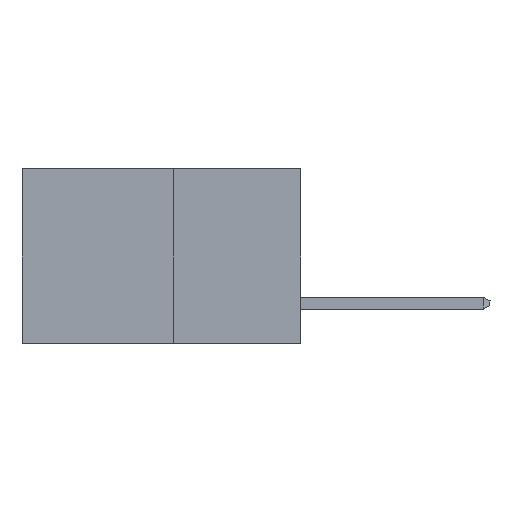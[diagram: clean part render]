
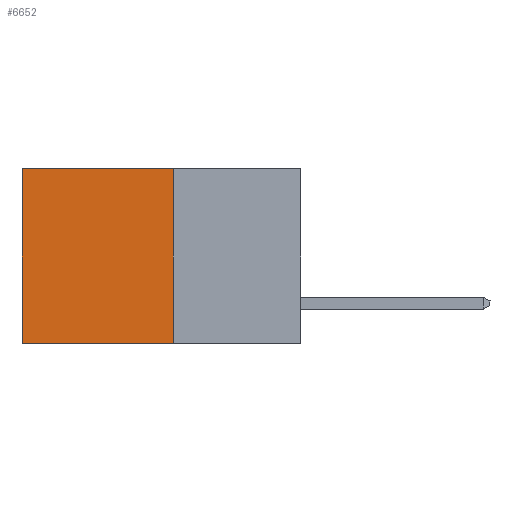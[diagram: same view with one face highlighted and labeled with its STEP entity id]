
A CAD part, left-side view. The second image highlights one B-rep face of the part: STEP entity #6652.
In plain terms, the highlighted planar face has unit normal (-1, 0, 0).
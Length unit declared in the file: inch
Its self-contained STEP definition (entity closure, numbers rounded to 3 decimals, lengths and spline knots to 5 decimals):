
#499 = ORIENTED_EDGE ( 'NONE', *, *, #7842, .T. ) ;
#1290 = DIRECTION ( 'NONE',  ( 0., 0., -1. ) ) ;
#1353 = EDGE_LOOP ( 'NONE', ( #499, #7801, #4283, #7589 ) ) ;
#1974 = LINE ( 'NONE', #6457, #2198 ) ;
#2198 = VECTOR ( 'NONE', #8405, 39.37008 ) ;
#2236 = DIRECTION ( 'NONE',  ( 1., 0., 0. ) ) ;
#2312 = DIRECTION ( 'NONE',  ( 0., 0., -1. ) ) ;
#2351 = LINE ( 'NONE', #6739, #5914 ) ;
#2553 = FACE_OUTER_BOUND ( 'NONE', #1353, .T. ) ;
#2642 = LINE ( 'NONE', #7510, #4272 ) ;
#3266 = EDGE_CURVE ( 'NONE', #6267, #3683, #5789, .T. ) ;
#3385 = CARTESIAN_POINT ( 'NONE',  ( 0.277, 0.59, -0.37 ) ) ;
#3669 = EDGE_CURVE ( 'NONE', #3683, #6469, #1974, .T. ) ;
#3683 = VERTEX_POINT ( 'NONE', #6424 ) ;
#4036 = VECTOR ( 'NONE', #1290, 39.37008 ) ;
#4272 = VECTOR ( 'NONE', #4903, 39.37008 ) ;
#4283 = ORIENTED_EDGE ( 'NONE', *, *, #3266, .F. ) ;
#4903 = DIRECTION ( 'NONE',  ( 0., 0., -1. ) ) ;
#5360 = AXIS2_PLACEMENT_3D ( 'NONE', #6224, #2236, #2312 ) ;
#5653 = CARTESIAN_POINT ( 'NONE',  ( 0.277, 0.27, -0.37 ) ) ;
#5789 = LINE ( 'NONE', #5653, #4036 ) ;
#5914 = VECTOR ( 'NONE', #6766, 39.37008 ) ;
#6224 = CARTESIAN_POINT ( 'NONE',  ( 0.277, 0.27, -0.37 ) ) ;
#6267 = VERTEX_POINT ( 'NONE', #7717 ) ;
#6354 = CARTESIAN_POINT ( 'NONE',  ( 0.277, 0.59, 0. ) ) ;
#6383 = VERTEX_POINT ( 'NONE', #6354 ) ;
#6424 = CARTESIAN_POINT ( 'NONE',  ( 0.277, 0.27, -0.37 ) ) ;
#6457 = CARTESIAN_POINT ( 'NONE',  ( 0.277, 0.27, -0.37 ) ) ;
#6469 = VERTEX_POINT ( 'NONE', #3385 ) ;
#6645 = PLANE ( 'NONE',  #5360 ) ;
#6652 = ADVANCED_FACE ( 'NONE', ( #2553 ), #6645, .F. ) ;
#6739 = CARTESIAN_POINT ( 'NONE',  ( 0.277, 0.27, 0. ) ) ;
#6766 = DIRECTION ( 'NONE',  ( 0., 1., 0. ) ) ;
#7510 = CARTESIAN_POINT ( 'NONE',  ( 0.277, 0.59, -0.37 ) ) ;
#7589 = ORIENTED_EDGE ( 'NONE', *, *, #8526, .T. ) ;
#7717 = CARTESIAN_POINT ( 'NONE',  ( 0.277, 0.27, 0. ) ) ;
#7801 = ORIENTED_EDGE ( 'NONE', *, *, #3669, .F. ) ;
#7842 = EDGE_CURVE ( 'NONE', #6383, #6469, #2642, .T. ) ;
#8405 = DIRECTION ( 'NONE',  ( 0., 1., 0. ) ) ;
#8526 = EDGE_CURVE ( 'NONE', #6267, #6383, #2351, .T. ) ;
